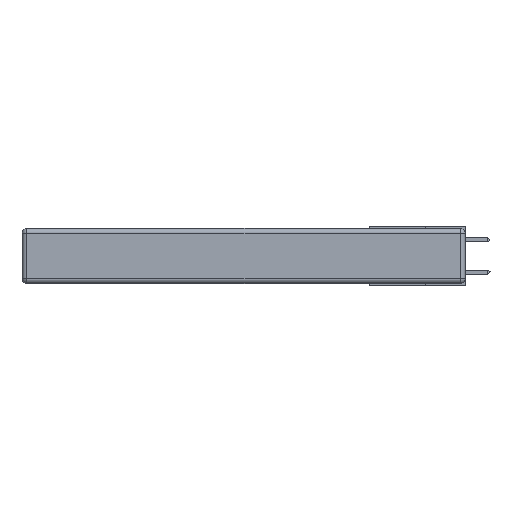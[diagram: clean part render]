
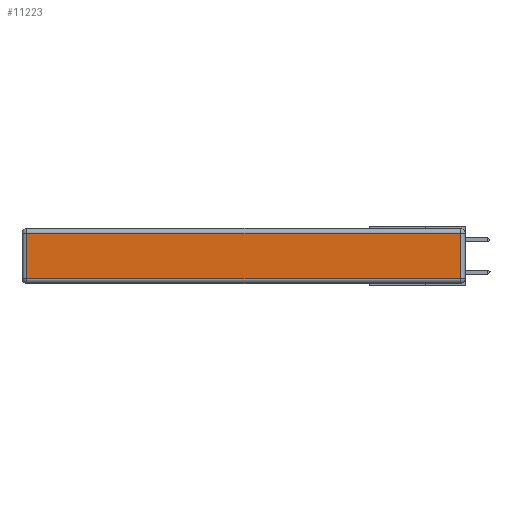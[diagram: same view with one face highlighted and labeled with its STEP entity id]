
A CAD part, left-side view. The second image highlights one B-rep face of the part: STEP entity #11223.
In plain terms, the highlighted planar face has unit normal (-1, 0, 0).
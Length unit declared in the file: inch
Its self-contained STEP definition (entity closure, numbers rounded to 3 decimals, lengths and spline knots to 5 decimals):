
#344 = VERTEX_POINT ( 'NONE', #6107 ) ;
#396 = EDGE_CURVE ( 'NONE', #7778, #344, #2959, .T. ) ;
#401 = DIRECTION ( 'NONE',  ( 0., 0., 1. ) ) ;
#527 = VERTEX_POINT ( 'NONE', #9130 ) ;
#1107 = CARTESIAN_POINT ( 'NONE',  ( 0., 2.72, -0.343 ) ) ;
#1708 = VECTOR ( 'NONE', #6061, 39.37008 ) ;
#1962 = VERTEX_POINT ( 'NONE', #11909 ) ;
#2350 = CARTESIAN_POINT ( 'NONE',  ( 0., 2.72, -0.03 ) ) ;
#2354 = LINE ( 'NONE', #5681, #10168 ) ;
#2392 = CARTESIAN_POINT ( 'NONE',  ( 0., 0., -0.343 ) ) ;
#2959 = LINE ( 'NONE', #1107, #8934 ) ;
#3142 = CARTESIAN_POINT ( 'NONE',  ( 0., 0., -0.313 ) ) ;
#4259 = EDGE_CURVE ( 'NONE', #527, #1962, #11016, .T. ) ;
#4635 = FACE_OUTER_BOUND ( 'NONE', #6736, .T. ) ;
#5305 = CARTESIAN_POINT ( 'NONE',  ( 0., 0.03, -0.343 ) ) ;
#5338 = DIRECTION ( 'NONE',  ( -1., 0., 0. ) ) ;
#5681 = CARTESIAN_POINT ( 'NONE',  ( 0., 2.75, -0.03 ) ) ;
#6061 = DIRECTION ( 'NONE',  ( 0., -1., 0. ) ) ;
#6107 = CARTESIAN_POINT ( 'NONE',  ( 0., 2.72, -0.313 ) ) ;
#6736 = EDGE_LOOP ( 'NONE', ( #9285, #10756, #8666, #7622 ) ) ;
#7622 = ORIENTED_EDGE ( 'NONE', *, *, #396, .T. ) ;
#7628 = DIRECTION ( 'NONE',  ( 0., 1., 0. ) ) ;
#7778 = VERTEX_POINT ( 'NONE', #2350 ) ;
#8040 = EDGE_CURVE ( 'NONE', #1962, #7778, #2354, .T. ) ;
#8083 = VECTOR ( 'NONE', #401, 39.37008 ) ;
#8159 = LINE ( 'NONE', #3142, #1708 ) ;
#8200 = EDGE_CURVE ( 'NONE', #344, #527, #8159, .T. ) ;
#8666 = ORIENTED_EDGE ( 'NONE', *, *, #8040, .T. ) ;
#8934 = VECTOR ( 'NONE', #11040, 39.37008 ) ;
#9130 = CARTESIAN_POINT ( 'NONE',  ( 0., 0.03, -0.313 ) ) ;
#9285 = ORIENTED_EDGE ( 'NONE', *, *, #8200, .T. ) ;
#10168 = VECTOR ( 'NONE', #7628, 39.37008 ) ;
#10555 = AXIS2_PLACEMENT_3D ( 'NONE', #2392, #5338, #12219 ) ;
#10756 = ORIENTED_EDGE ( 'NONE', *, *, #4259, .T. ) ;
#11016 = LINE ( 'NONE', #5305, #8083 ) ;
#11040 = DIRECTION ( 'NONE',  ( 0., 0., -1. ) ) ;
#11223 = ADVANCED_FACE ( 'NONE', ( #4635 ), #12147, .T. ) ;
#11909 = CARTESIAN_POINT ( 'NONE',  ( 0., 0.03, -0.03 ) ) ;
#12147 = PLANE ( 'NONE',  #10555 ) ;
#12219 = DIRECTION ( 'NONE',  ( 0., 0., 1. ) ) ;
